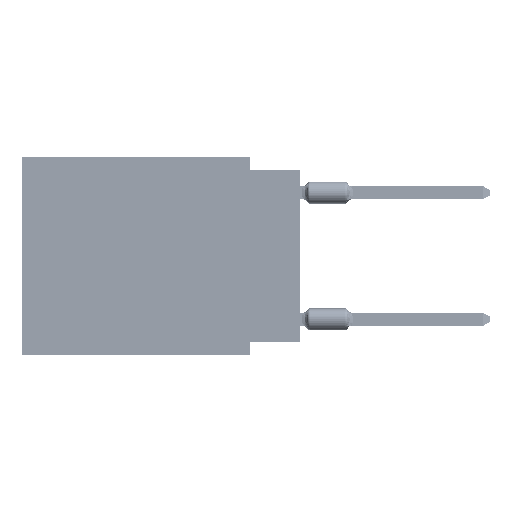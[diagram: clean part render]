
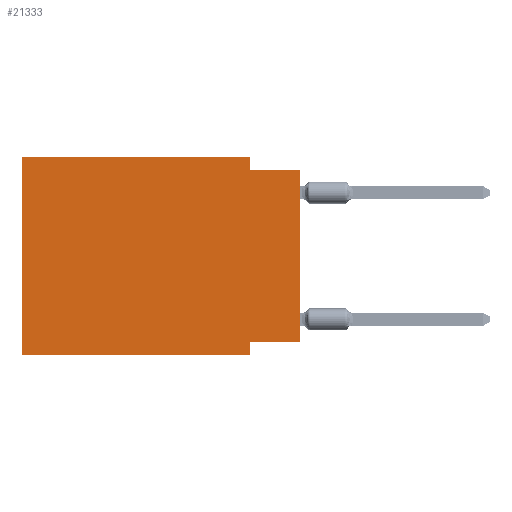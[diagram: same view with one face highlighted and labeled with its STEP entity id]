
A CAD part, left-side view. The second image highlights one B-rep face of the part: STEP entity #21333.
In plain terms, the highlighted planar face has unit normal (-1, 0, 0).
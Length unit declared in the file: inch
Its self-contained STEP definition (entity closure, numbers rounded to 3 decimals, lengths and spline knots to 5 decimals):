
#183 = VERTEX_POINT ( 'NONE', #75283 ) ;
#404 = ORIENTED_EDGE ( 'NONE', *, *, #39021, .F. ) ;
#632 = VERTEX_POINT ( 'NONE', #16050 ) ;
#671 = CARTESIAN_POINT ( 'NONE',  ( 0., 0.1, 0. ) ) ;
#1056 = DIRECTION ( 'NONE',  ( 0., 0., -1. ) ) ;
#1189 = DIRECTION ( 'NONE',  ( 0., 1., 0. ) ) ;
#1537 = FACE_OUTER_BOUND ( 'NONE', #72817, .T. ) ;
#4597 = DIRECTION ( 'NONE',  ( 0., -1., 0. ) ) ;
#5298 = VERTEX_POINT ( 'NONE', #72014 ) ;
#5689 = CARTESIAN_POINT ( 'NONE',  ( 0., 0.1, -0.39 ) ) ;
#5938 = VERTEX_POINT ( 'NONE', #40427 ) ;
#7542 = ORIENTED_EDGE ( 'NONE', *, *, #34088, .F. ) ;
#8667 = VECTOR ( 'NONE', #1189, 39.37008 ) ;
#11163 = CARTESIAN_POINT ( 'NONE',  ( 0., 0.1, -0.39 ) ) ;
#11239 = CARTESIAN_POINT ( 'NONE',  ( 0., 0.55, 0. ) ) ;
#12091 = EDGE_CURVE ( 'NONE', #65535, #72652, #61906, .T. ) ;
#12734 = CARTESIAN_POINT ( 'NONE',  ( 0., 0., -0.025 ) ) ;
#12979 = ORIENTED_EDGE ( 'NONE', *, *, #61683, .T. ) ;
#14933 = CARTESIAN_POINT ( 'NONE',  ( 0., 0.55, 0. ) ) ;
#16050 = CARTESIAN_POINT ( 'NONE',  ( 0., 0.1, 0. ) ) ;
#16454 = VECTOR ( 'NONE', #1056, 39.37008 ) ;
#16796 = ORIENTED_EDGE ( 'NONE', *, *, #61948, .F. ) ;
#18224 = CARTESIAN_POINT ( 'NONE',  ( 0., 0., -0.365 ) ) ;
#19165 = VERTEX_POINT ( 'NONE', #18224 ) ;
#19420 = VECTOR ( 'NONE', #32192, 39.37008 ) ;
#19476 = LINE ( 'NONE', #671, #16454 ) ;
#20938 = VECTOR ( 'NONE', #63696, 39.37008 ) ;
#21333 = ADVANCED_FACE ( 'NONE', ( #1537 ), #37989, .F. ) ;
#22251 = DIRECTION ( 'NONE',  ( 0., 0., 1. ) ) ;
#28508 = CARTESIAN_POINT ( 'NONE',  ( 0., 0., 0. ) ) ;
#28992 = ORIENTED_EDGE ( 'NONE', *, *, #12091, .T. ) ;
#29585 = EDGE_CURVE ( 'NONE', #5298, #632, #59051, .T. ) ;
#31673 = CARTESIAN_POINT ( 'NONE',  ( 0., 0.55, -0.39 ) ) ;
#32192 = DIRECTION ( 'NONE',  ( 0., 0., 1. ) ) ;
#32294 = LINE ( 'NONE', #56581, #38060 ) ;
#33337 = LINE ( 'NONE', #14933, #19420 ) ;
#34088 = EDGE_CURVE ( 'NONE', #5938, #72652, #59368, .T. ) ;
#34734 = ORIENTED_EDGE ( 'NONE', *, *, #53573, .F. ) ;
#37636 = CARTESIAN_POINT ( 'NONE',  ( 0., 0., -0.365 ) ) ;
#37989 = PLANE ( 'NONE',  #38844 ) ;
#38060 = VECTOR ( 'NONE', #76395, 39.37008 ) ;
#38844 = AXIS2_PLACEMENT_3D ( 'NONE', #62643, #62286, #48972 ) ;
#39021 = EDGE_CURVE ( 'NONE', #632, #183, #19476, .T. ) ;
#40427 = CARTESIAN_POINT ( 'NONE',  ( 0., 0.1, -0.365 ) ) ;
#43377 = EDGE_CURVE ( 'NONE', #65535, #5298, #33337, .T. ) ;
#43527 = CARTESIAN_POINT ( 'NONE',  ( 0., 0.55, -0.39 ) ) ;
#43910 = LINE ( 'NONE', #37636, #8667 ) ;
#48972 = DIRECTION ( 'NONE',  ( 0., 0., -1. ) ) ;
#51224 = VECTOR ( 'NONE', #22251, 39.37008 ) ;
#52043 = LINE ( 'NONE', #28508, #51224 ) ;
#53448 = VERTEX_POINT ( 'NONE', #12734 ) ;
#53573 = EDGE_CURVE ( 'NONE', #183, #53448, #32294, .T. ) ;
#55258 = DIRECTION ( 'NONE',  ( 0., -1., 0. ) ) ;
#56581 = CARTESIAN_POINT ( 'NONE',  ( 0., 0., -0.025 ) ) ;
#59051 = LINE ( 'NONE', #11239, #68196 ) ;
#59368 = LINE ( 'NONE', #5689, #20938 ) ;
#61683 = EDGE_CURVE ( 'NONE', #19165, #53448, #52043, .T. ) ;
#61906 = LINE ( 'NONE', #43527, #70736 ) ;
#61948 = EDGE_CURVE ( 'NONE', #19165, #5938, #43910, .T. ) ;
#62286 = DIRECTION ( 'NONE',  ( 1., 0., 0. ) ) ;
#62643 = CARTESIAN_POINT ( 'NONE',  ( 0., 0.55, 0. ) ) ;
#63696 = DIRECTION ( 'NONE',  ( 0., 0., -1. ) ) ;
#65329 = ORIENTED_EDGE ( 'NONE', *, *, #43377, .F. ) ;
#65535 = VERTEX_POINT ( 'NONE', #31673 ) ;
#68196 = VECTOR ( 'NONE', #4597, 39.37008 ) ;
#68624 = ORIENTED_EDGE ( 'NONE', *, *, #29585, .F. ) ;
#70736 = VECTOR ( 'NONE', #55258, 39.37008 ) ;
#72014 = CARTESIAN_POINT ( 'NONE',  ( 0., 0.55, 0. ) ) ;
#72652 = VERTEX_POINT ( 'NONE', #11163 ) ;
#72817 = EDGE_LOOP ( 'NONE', ( #12979, #34734, #404, #68624, #65329, #28992, #7542, #16796 ) ) ;
#75283 = CARTESIAN_POINT ( 'NONE',  ( 0., 0.1, -0.025 ) ) ;
#76395 = DIRECTION ( 'NONE',  ( 0., -1., 0. ) ) ;
